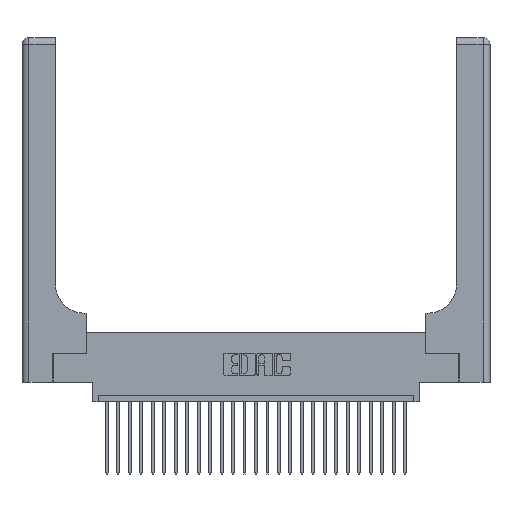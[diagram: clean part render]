
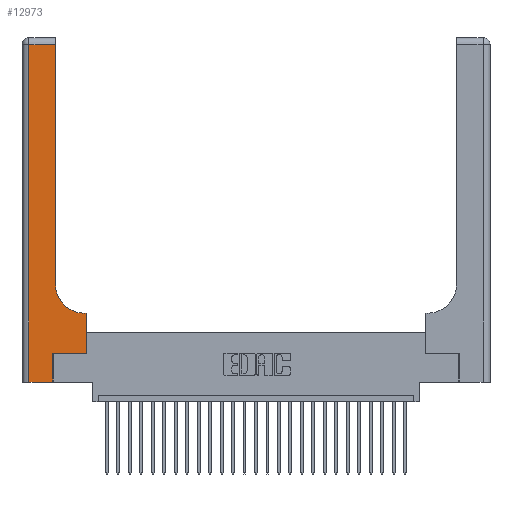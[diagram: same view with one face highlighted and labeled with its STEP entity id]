
A CAD part, top view. The second image highlights one B-rep face of the part: STEP entity #12973.
In plain terms, the highlighted planar face has unit normal (0, 0, 1).
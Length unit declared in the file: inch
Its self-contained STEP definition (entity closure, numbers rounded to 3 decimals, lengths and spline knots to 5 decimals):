
#782 = VECTOR ( 'NONE', #5875, 39.37008 ) ;
#990 = CARTESIAN_POINT ( 'NONE',  ( 0.5415, 0.85, 0.37 ) ) ;
#1020 = CARTESIAN_POINT ( 'NONE',  ( 0., 2.94, 0.37 ) ) ;
#1249 = CARTESIAN_POINT ( 'NONE',  ( 0.2915, 3., 0.37 ) ) ;
#1377 = ORIENTED_EDGE ( 'NONE', *, *, #3494, .T. ) ;
#1911 = VECTOR ( 'NONE', #12571, 39.37008 ) ;
#2148 = CARTESIAN_POINT ( 'NONE',  ( 0.06, 3., 0.37 ) ) ;
#2705 = ORIENTED_EDGE ( 'NONE', *, *, #9892, .T. ) ;
#2772 = VERTEX_POINT ( 'NONE', #15575 ) ;
#3434 = VECTOR ( 'NONE', #13315, 39.37008 ) ;
#3494 = EDGE_CURVE ( 'NONE', #19651, #13182, #10919, .T. ) ;
#3719 = CARTESIAN_POINT ( 'NONE',  ( 0., 3., 0.37 ) ) ;
#3851 = VECTOR ( 'NONE', #4866, 39.37008 ) ;
#4454 = DIRECTION ( 'NONE',  ( 0., 1., 0. ) ) ;
#4827 = CARTESIAN_POINT ( 'NONE',  ( 0.2915, 0.85, 0.37 ) ) ;
#4866 = DIRECTION ( 'NONE',  ( 1., 0., 0. ) ) ;
#5140 = PLANE ( 'NONE',  #14443 ) ;
#5191 = LINE ( 'NONE', #17591, #3851 ) ;
#5573 = VERTEX_POINT ( 'NONE', #25095 ) ;
#5875 = DIRECTION ( 'NONE',  ( 0., 1., 0. ) ) ;
#6485 = DIRECTION ( 'NONE',  ( 0., -1., 0. ) ) ;
#6873 = CARTESIAN_POINT ( 'NONE',  ( 0.269, 0., 0.37 ) ) ;
#7147 = CARTESIAN_POINT ( 'NONE',  ( 0.06, 2.94, 0.37 ) ) ;
#7180 = DIRECTION ( 'NONE',  ( 0., 0., -1. ) ) ;
#7348 = AXIS2_PLACEMENT_3D ( 'NONE', #990, #11820, #18035 ) ;
#7363 = VERTEX_POINT ( 'NONE', #12285 ) ;
#8093 = CARTESIAN_POINT ( 'NONE',  ( 0.2915, 0.6, 0.37 ) ) ;
#8253 = LINE ( 'NONE', #1020, #8582 ) ;
#8582 = VECTOR ( 'NONE', #9786, 39.37008 ) ;
#9757 = LINE ( 'NONE', #25952, #26094 ) ;
#9786 = DIRECTION ( 'NONE',  ( -1., 0., 0. ) ) ;
#9892 = EDGE_CURVE ( 'NONE', #10694, #16695, #13989, .T. ) ;
#10119 = CARTESIAN_POINT ( 'NONE',  ( 0.5415, 0.6, 0.37 ) ) ;
#10694 = VERTEX_POINT ( 'NONE', #15277 ) ;
#10919 = LINE ( 'NONE', #2148, #20205 ) ;
#11341 = CARTESIAN_POINT ( 'NONE',  ( 0.06, 0., 0.37 ) ) ;
#11779 = EDGE_CURVE ( 'NONE', #2772, #19651, #8253, .T. ) ;
#11820 = DIRECTION ( 'NONE',  ( 0., 0., -1. ) ) ;
#12285 = CARTESIAN_POINT ( 'NONE',  ( 0.269, 0.25, 0.37 ) ) ;
#12571 = DIRECTION ( 'NONE',  ( -1., 0., 0. ) ) ;
#12973 = ADVANCED_FACE ( 'NONE', ( #24168 ), #5140, .F. ) ;
#13182 = VERTEX_POINT ( 'NONE', #11341 ) ;
#13289 = VECTOR ( 'NONE', #4454, 39.37008 ) ;
#13315 = DIRECTION ( 'NONE',  ( 0., 1., 0. ) ) ;
#13925 = ORIENTED_EDGE ( 'NONE', *, *, #21477, .T. ) ;
#13989 = LINE ( 'NONE', #8093, #1911 ) ;
#14443 = AXIS2_PLACEMENT_3D ( 'NONE', #3719, #7180, #15501 ) ;
#15277 = CARTESIAN_POINT ( 'NONE',  ( 0.5585, 0.6, 0.37 ) ) ;
#15501 = DIRECTION ( 'NONE',  ( -1., 0., 0. ) ) ;
#15575 = CARTESIAN_POINT ( 'NONE',  ( 0.2915, 2.94, 0.37 ) ) ;
#15701 = VERTEX_POINT ( 'NONE', #4827 ) ;
#16173 = VERTEX_POINT ( 'NONE', #18198 ) ;
#16223 = ORIENTED_EDGE ( 'NONE', *, *, #18449, .T. ) ;
#16413 = EDGE_CURVE ( 'NONE', #16173, #7363, #25508, .T. ) ;
#16695 = VERTEX_POINT ( 'NONE', #10119 ) ;
#16928 = ORIENTED_EDGE ( 'NONE', *, *, #21911, .T. ) ;
#17247 = ORIENTED_EDGE ( 'NONE', *, *, #11779, .T. ) ;
#17591 = CARTESIAN_POINT ( 'NONE',  ( 0.269, 0.25, 0.37 ) ) ;
#18035 = DIRECTION ( 'NONE',  ( 1., 0., 0. ) ) ;
#18198 = CARTESIAN_POINT ( 'NONE',  ( 0.269, 0., 0.37 ) ) ;
#18420 = ORIENTED_EDGE ( 'NONE', *, *, #25674, .T. ) ;
#18449 = EDGE_CURVE ( 'NONE', #16695, #15701, #24750, .T. ) ;
#19651 = VERTEX_POINT ( 'NONE', #7147 ) ;
#20205 = VECTOR ( 'NONE', #6485, 39.37008 ) ;
#20729 = EDGE_CURVE ( 'NONE', #5573, #10694, #24273, .T. ) ;
#20749 = EDGE_LOOP ( 'NONE', ( #16928, #17247, #1377, #18420, #26129, #13925, #21409, #2705, #16223 ) ) ;
#21409 = ORIENTED_EDGE ( 'NONE', *, *, #20729, .T. ) ;
#21477 = EDGE_CURVE ( 'NONE', #7363, #5573, #5191, .T. ) ;
#21911 = EDGE_CURVE ( 'NONE', #15701, #2772, #25898, .T. ) ;
#23409 = CARTESIAN_POINT ( 'NONE',  ( 0.5585, 0.25, 0.37 ) ) ;
#24000 = DIRECTION ( 'NONE',  ( 1., 0., 0. ) ) ;
#24168 = FACE_OUTER_BOUND ( 'NONE', #20749, .T. ) ;
#24273 = LINE ( 'NONE', #23409, #13289 ) ;
#24750 = CIRCLE ( 'NONE', #7348, 0.25 ) ;
#25095 = CARTESIAN_POINT ( 'NONE',  ( 0.5585, 0.25, 0.37 ) ) ;
#25508 = LINE ( 'NONE', #6873, #3434 ) ;
#25674 = EDGE_CURVE ( 'NONE', #13182, #16173, #9757, .T. ) ;
#25898 = LINE ( 'NONE', #1249, #782 ) ;
#25952 = CARTESIAN_POINT ( 'NONE',  ( 0., 0., 0.37 ) ) ;
#26094 = VECTOR ( 'NONE', #24000, 39.37008 ) ;
#26129 = ORIENTED_EDGE ( 'NONE', *, *, #16413, .T. ) ;
